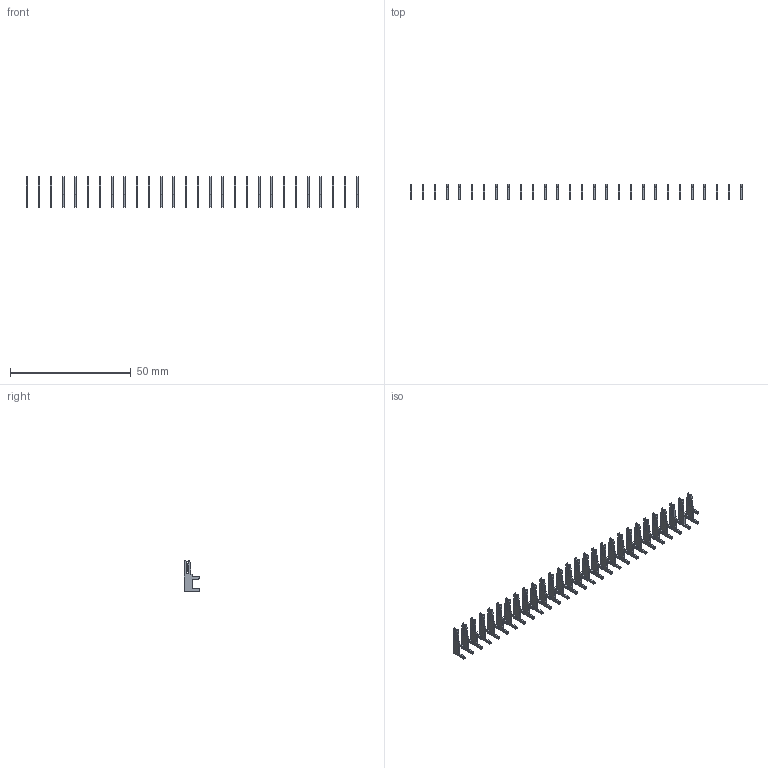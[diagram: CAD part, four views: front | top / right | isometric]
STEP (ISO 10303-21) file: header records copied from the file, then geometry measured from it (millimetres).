
FILE_DESCRIPTION (( 'STEP AP203' ), '1' );
FILE_NAME ('105-028-203-200.STEP', '2020-08-29T23:39:29', ( '' ), ( '' ), 'SwSTEP 2.0', 'SolidWorks 2020', '' );
FILE_SCHEMA (( 'CONFIG_CONTROL_DESIGN' ));
Length unit declared in the file: inch
Products named in the file (2): 100-290-001_100-290-203; 105-028-203-200
Assembly tree (28 placements, depth 2):
  105-028-203-200
    100-290-001_100-290-203  x28
Bounding box: 137.76 x 6.53 x 12.7 mm (x, y, z)
Volume: 706.9 mm3; surface area: 3240.1 mm2
Topology: 28 solids, 28 shells, 784 faces, 2184 edges, 1456 vertices
Faces by surface type: plane 588, cylinder 196
Entity records: 1960 total; most frequent: DIRECTION 206, CARTESIAN_POINT 201, ORIENTED_EDGE 156, EDGE_CURVE 78, AXIS2_PLACEMENT_3D 73, CALENDAR_DATE 66, DATE_AND_TIME 66, LOCAL_TIME 66
